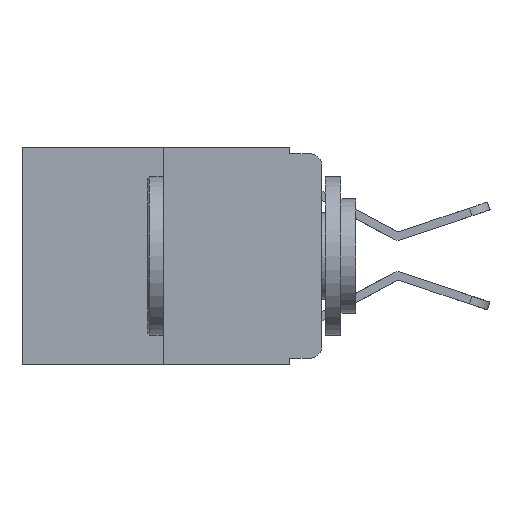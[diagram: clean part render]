
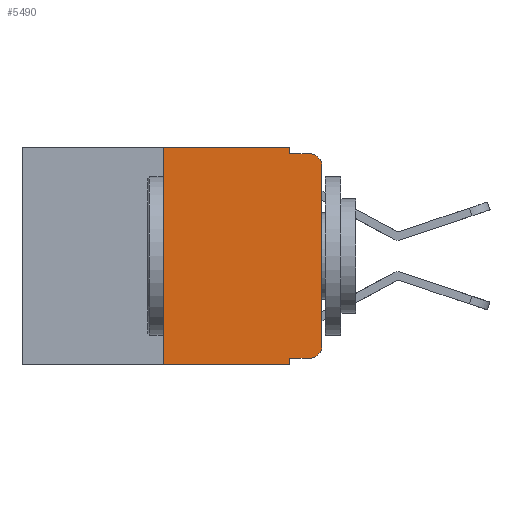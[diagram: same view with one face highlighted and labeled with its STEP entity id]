
A CAD part, left-side view. The second image highlights one B-rep face of the part: STEP entity #5490.
In plain terms, the highlighted planar face has unit normal (-1, 0, 0).
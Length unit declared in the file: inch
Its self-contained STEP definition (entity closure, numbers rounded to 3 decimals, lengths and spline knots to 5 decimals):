
#101 = LINE ( 'NONE', #11598, #15020 ) ;
#297 = VECTOR ( 'NONE', #4395, 39.37008 ) ;
#586 = ORIENTED_EDGE ( 'NONE', *, *, #8818, .F. ) ;
#613 = DIRECTION ( 'NONE',  ( -1., 0., 0. ) ) ;
#677 = PLANE ( 'NONE',  #2993 ) ;
#990 = LINE ( 'NONE', #18087, #15821 ) ;
#1118 = LINE ( 'NONE', #16311, #15946 ) ;
#1644 = LINE ( 'NONE', #7053, #9032 ) ;
#1859 = EDGE_CURVE ( 'NONE', #9056, #4821, #990, .T. ) ;
#2025 = DIRECTION ( 'NONE',  ( 0., 0., 1. ) ) ;
#2079 = VECTOR ( 'NONE', #2025, 39.37008 ) ;
#2210 = DIRECTION ( 'NONE',  ( 1., 0., 0. ) ) ;
#2240 = CARTESIAN_POINT ( 'NONE',  ( 0., 0.051, -0.01 ) ) ;
#2993 = AXIS2_PLACEMENT_3D ( 'NONE', #3838, #2210, #9336 ) ;
#3221 = CARTESIAN_POINT ( 'NONE',  ( 0., 0.25, -0.343 ) ) ;
#3580 = DIRECTION ( 'NONE',  ( 0., 0., -1. ) ) ;
#3838 = CARTESIAN_POINT ( 'NONE',  ( 0., 0.473, 0. ) ) ;
#3888 = VERTEX_POINT ( 'NONE', #15808 ) ;
#4070 = DIRECTION ( 'NONE',  ( -1., 0., 0. ) ) ;
#4395 = DIRECTION ( 'NONE',  ( 0., -1., 0. ) ) ;
#4821 = VERTEX_POINT ( 'NONE', #15586 ) ;
#4871 = EDGE_CURVE ( 'NONE', #16337, #9589, #101, .T. ) ;
#5041 = CARTESIAN_POINT ( 'NONE',  ( 0., 0., 0. ) ) ;
#5266 = CARTESIAN_POINT ( 'NONE',  ( 0., 0., -0.313 ) ) ;
#5366 = ORIENTED_EDGE ( 'NONE', *, *, #4871, .F. ) ;
#5490 = ADVANCED_FACE ( 'NONE', ( #9126 ), #677, .F. ) ;
#5669 = LINE ( 'NONE', #2240, #12790 ) ;
#5898 = CARTESIAN_POINT ( 'NONE',  ( 0., 0.473, -0.343 ) ) ;
#6230 = VERTEX_POINT ( 'NONE', #5266 ) ;
#6837 = EDGE_CURVE ( 'NONE', #9589, #3888, #5669, .T. ) ;
#7053 = CARTESIAN_POINT ( 'NONE',  ( 0., 0.473, 0. ) ) ;
#7261 = DIRECTION ( 'NONE',  ( 0., 0., -1. ) ) ;
#7502 = VECTOR ( 'NONE', #11374, 39.37008 ) ;
#8045 = ORIENTED_EDGE ( 'NONE', *, *, #14729, .T. ) ;
#8258 = CIRCLE ( 'NONE', #12395, 0.02 ) ;
#8559 = ORIENTED_EDGE ( 'NONE', *, *, #8783, .T. ) ;
#8718 = VERTEX_POINT ( 'NONE', #13799 ) ;
#8783 = EDGE_CURVE ( 'NONE', #8718, #3888, #17299, .T. ) ;
#8818 = EDGE_CURVE ( 'NONE', #4821, #16337, #1644, .T. ) ;
#8937 = ORIENTED_EDGE ( 'NONE', *, *, #1859, .F. ) ;
#9032 = VECTOR ( 'NONE', #18319, 39.37008 ) ;
#9056 = VERTEX_POINT ( 'NONE', #3221 ) ;
#9126 = FACE_OUTER_BOUND ( 'NONE', #11529, .T. ) ;
#9336 = DIRECTION ( 'NONE',  ( 0., 0., -1. ) ) ;
#9461 = CARTESIAN_POINT ( 'NONE',  ( 0., 0.02, -0.313 ) ) ;
#9589 = VERTEX_POINT ( 'NONE', #11617 ) ;
#9729 = EDGE_CURVE ( 'NONE', #6230, #8718, #12277, .T. ) ;
#9973 = CARTESIAN_POINT ( 'NONE',  ( 0., 0.051, -0.333 ) ) ;
#10894 = DIRECTION ( 'NONE',  ( 0., 0., -1. ) ) ;
#11059 = DIRECTION ( 'NONE',  ( 0., 0., 1. ) ) ;
#11101 = LINE ( 'NONE', #5898, #297 ) ;
#11288 = LINE ( 'NONE', #9973, #7502 ) ;
#11374 = DIRECTION ( 'NONE',  ( 0., -1., 0. ) ) ;
#11529 = EDGE_LOOP ( 'NONE', ( #12494, #8559, #18154, #5366, #586, #8937, #11802, #17200, #8045, #17484 ) ) ;
#11558 = CARTESIAN_POINT ( 'NONE',  ( 0., 0.02, -0.333 ) ) ;
#11598 = CARTESIAN_POINT ( 'NONE',  ( 0., 0.051, 0. ) ) ;
#11617 = CARTESIAN_POINT ( 'NONE',  ( 0., 0.051, -0.01 ) ) ;
#11802 = ORIENTED_EDGE ( 'NONE', *, *, #13689, .T. ) ;
#12003 = AXIS2_PLACEMENT_3D ( 'NONE', #12672, #4070, #14049 ) ;
#12277 = LINE ( 'NONE', #5041, #2079 ) ;
#12395 = AXIS2_PLACEMENT_3D ( 'NONE', #9461, #613, #10894 ) ;
#12494 = ORIENTED_EDGE ( 'NONE', *, *, #9729, .T. ) ;
#12588 = VERTEX_POINT ( 'NONE', #15724 ) ;
#12672 = CARTESIAN_POINT ( 'NONE',  ( 0., 0.02, -0.03 ) ) ;
#12790 = VECTOR ( 'NONE', #13677, 39.37008 ) ;
#12875 = EDGE_CURVE ( 'NONE', #17555, #6230, #8258, .T. ) ;
#13407 = CARTESIAN_POINT ( 'NONE',  ( 0., 0.051, -0.333 ) ) ;
#13677 = DIRECTION ( 'NONE',  ( 0., -1., 0. ) ) ;
#13689 = EDGE_CURVE ( 'NONE', #9056, #12588, #11101, .T. ) ;
#13735 = CARTESIAN_POINT ( 'NONE',  ( 0., 0.051, 0. ) ) ;
#13799 = CARTESIAN_POINT ( 'NONE',  ( 0., 0., -0.03 ) ) ;
#14049 = DIRECTION ( 'NONE',  ( 0., 0., -1. ) ) ;
#14729 = EDGE_CURVE ( 'NONE', #16801, #17555, #11288, .T. ) ;
#15020 = VECTOR ( 'NONE', #7261, 39.37008 ) ;
#15586 = CARTESIAN_POINT ( 'NONE',  ( 0., 0.25, 0. ) ) ;
#15724 = CARTESIAN_POINT ( 'NONE',  ( 0., 0.051, -0.343 ) ) ;
#15808 = CARTESIAN_POINT ( 'NONE',  ( 0., 0.02, -0.01 ) ) ;
#15821 = VECTOR ( 'NONE', #11059, 39.37008 ) ;
#15946 = VECTOR ( 'NONE', #3580, 39.37008 ) ;
#16311 = CARTESIAN_POINT ( 'NONE',  ( 0., 0.051, 0. ) ) ;
#16337 = VERTEX_POINT ( 'NONE', #13735 ) ;
#16801 = VERTEX_POINT ( 'NONE', #13407 ) ;
#17200 = ORIENTED_EDGE ( 'NONE', *, *, #18480, .F. ) ;
#17299 = CIRCLE ( 'NONE', #12003, 0.02 ) ;
#17484 = ORIENTED_EDGE ( 'NONE', *, *, #12875, .T. ) ;
#17555 = VERTEX_POINT ( 'NONE', #11558 ) ;
#18087 = CARTESIAN_POINT ( 'NONE',  ( 0., 0.25, 0. ) ) ;
#18154 = ORIENTED_EDGE ( 'NONE', *, *, #6837, .F. ) ;
#18319 = DIRECTION ( 'NONE',  ( 0., -1., 0. ) ) ;
#18480 = EDGE_CURVE ( 'NONE', #16801, #12588, #1118, .T. ) ;
